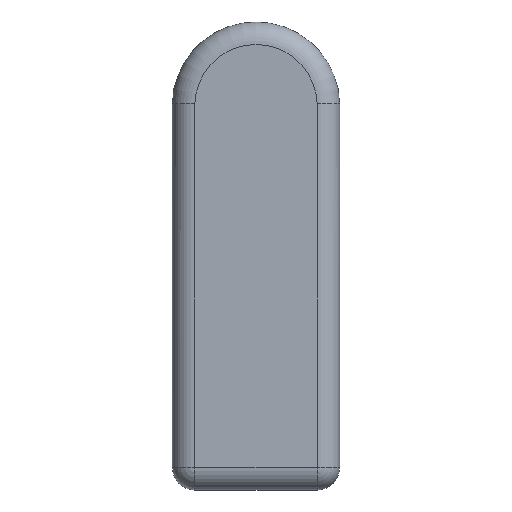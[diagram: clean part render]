
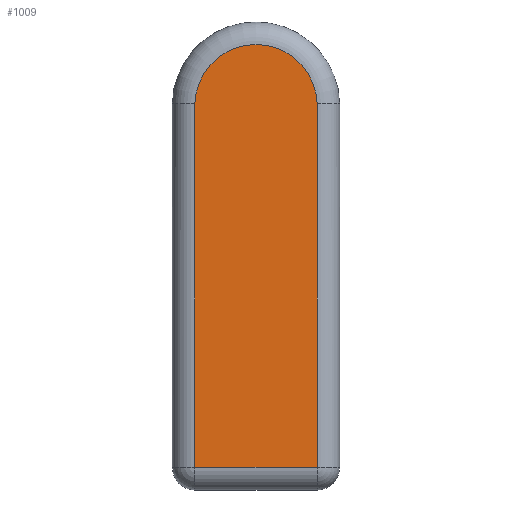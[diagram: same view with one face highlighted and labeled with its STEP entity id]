
A CAD part, top view. The second image highlights one B-rep face of the part: STEP entity #1009.
In plain terms, the highlighted planar face has unit normal (0, 0, 1).
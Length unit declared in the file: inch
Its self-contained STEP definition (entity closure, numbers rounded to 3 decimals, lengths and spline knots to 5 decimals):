
#1 = EDGE_CURVE ( 'NONE', #1332, #107, #1090, .T. ) ;
#76 = ORIENTED_EDGE ( 'NONE', *, *, #1, .T. ) ;
#107 = VERTEX_POINT ( 'NONE', #1219 ) ;
#129 = AXIS2_PLACEMENT_3D ( 'NONE', #333, #1072, #444 ) ;
#133 = VECTOR ( 'NONE', #1302, 39.37008 ) ;
#142 = CIRCLE ( 'NONE', #129, 0.53445 ) ;
#244 = VERTEX_POINT ( 'NONE', #842 ) ;
#333 = CARTESIAN_POINT ( 'NONE',  ( -0.03705, 1.30755, 0.25 ) ) ;
#359 = EDGE_CURVE ( 'NONE', #107, #244, #979, .T. ) ;
#362 = DIRECTION ( 'NONE',  ( 0., -1., 0. ) ) ;
#363 = EDGE_LOOP ( 'NONE', ( #387, #76, #461, #511 ) ) ;
#387 = ORIENTED_EDGE ( 'NONE', *, *, #949, .T. ) ;
#407 = LINE ( 'NONE', #988, #133 ) ;
#444 = DIRECTION ( 'NONE',  ( 1., 0., 0. ) ) ;
#454 = DIRECTION ( 'NONE',  ( 1., 0., 0. ) ) ;
#461 = ORIENTED_EDGE ( 'NONE', *, *, #359, .T. ) ;
#473 = CARTESIAN_POINT ( 'NONE',  ( -0.57117, -1.85258, 0.25 ) ) ;
#511 = ORIENTED_EDGE ( 'NONE', *, *, #712, .T. ) ;
#545 = CARTESIAN_POINT ( 'NONE',  ( 0.49707, -1.85258, 0.25 ) ) ;
#663 = CARTESIAN_POINT ( 'NONE',  ( 0.49707, -1.85258, 0.25 ) ) ;
#702 = VECTOR ( 'NONE', #971, 39.37008 ) ;
#712 = EDGE_CURVE ( 'NONE', #244, #948, #407, .T. ) ;
#757 = CARTESIAN_POINT ( 'NONE',  ( 0.49707, 1.32634, 0.25 ) ) ;
#765 = AXIS2_PLACEMENT_3D ( 'NONE', #663, #1084, #454 ) ;
#812 = CARTESIAN_POINT ( 'NONE',  ( -0.57117, 1.32634, 0.25 ) ) ;
#814 = VECTOR ( 'NONE', #362, 39.37008 ) ;
#842 = CARTESIAN_POINT ( 'NONE',  ( 0.49707, -1.85258, 0.25 ) ) ;
#866 = PLANE ( 'NONE',  #765 ) ;
#884 = FACE_OUTER_BOUND ( 'NONE', #363, .T. ) ;
#948 = VERTEX_POINT ( 'NONE', #757 ) ;
#949 = EDGE_CURVE ( 'NONE', #948, #1332, #142, .T. ) ;
#971 = DIRECTION ( 'NONE',  ( 1., 0., 0. ) ) ;
#979 = LINE ( 'NONE', #545, #702 ) ;
#988 = CARTESIAN_POINT ( 'NONE',  ( 0.49707, 1.32953, 0.25 ) ) ;
#1009 = ADVANCED_FACE ( 'NONE', ( #884 ), #866, .T. ) ;
#1072 = DIRECTION ( 'NONE',  ( 0., 0., 1. ) ) ;
#1084 = DIRECTION ( 'NONE',  ( 0., 0., 1. ) ) ;
#1090 = LINE ( 'NONE', #473, #814 ) ;
#1219 = CARTESIAN_POINT ( 'NONE',  ( -0.57117, -1.85258, 0.25 ) ) ;
#1302 = DIRECTION ( 'NONE',  ( 0., 1., 0. ) ) ;
#1332 = VERTEX_POINT ( 'NONE', #812 ) ;
